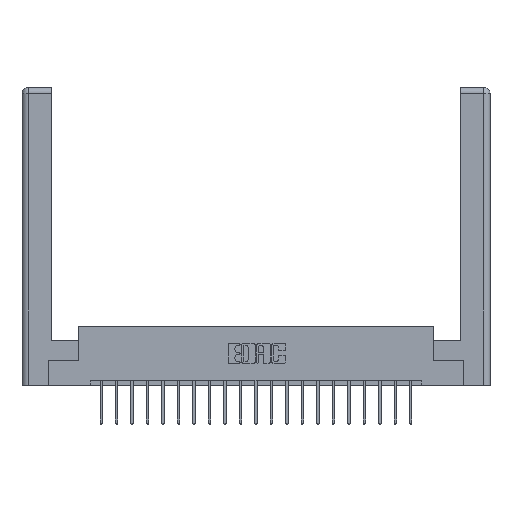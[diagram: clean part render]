
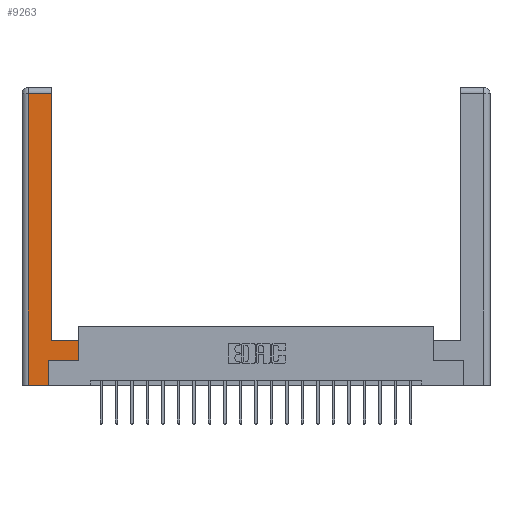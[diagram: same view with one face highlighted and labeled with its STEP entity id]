
A CAD part, top view. The second image highlights one B-rep face of the part: STEP entity #9263.
In plain terms, the highlighted planar face has unit normal (0, 0, 1).
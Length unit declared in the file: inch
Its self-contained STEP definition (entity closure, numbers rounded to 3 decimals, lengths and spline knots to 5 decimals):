
#172 = VECTOR ( 'NONE', #19106, 39.37008 ) ;
#198 = VECTOR ( 'NONE', #21235, 39.37008 ) ;
#546 = CARTESIAN_POINT ( 'NONE',  ( 0.565, 0.45, 0. ) ) ;
#695 = VECTOR ( 'NONE', #6751, 39.37008 ) ;
#976 = CARTESIAN_POINT ( 'NONE',  ( 0.265, 0., 0. ) ) ;
#1071 = CARTESIAN_POINT ( 'NONE',  ( 0.265, 0.245, 0. ) ) ;
#1499 = ORIENTED_EDGE ( 'NONE', *, *, #1673, .T. ) ;
#1673 = EDGE_CURVE ( 'NONE', #5320, #14640, #13986, .T. ) ;
#1814 = ORIENTED_EDGE ( 'NONE', *, *, #2555, .T. ) ;
#2351 = CARTESIAN_POINT ( 'NONE',  ( 0.0615, 0., 0. ) ) ;
#2555 = EDGE_CURVE ( 'NONE', #11462, #7162, #8593, .T. ) ;
#3026 = ORIENTED_EDGE ( 'NONE', *, *, #10543, .T. ) ;
#3735 = LINE ( 'NONE', #19542, #17870 ) ;
#4476 = DIRECTION ( 'NONE',  ( 1., 0., 0. ) ) ;
#5158 = CARTESIAN_POINT ( 'NONE',  ( 0.295, 0.45, 0. ) ) ;
#5320 = VERTEX_POINT ( 'NONE', #20268 ) ;
#5888 = PLANE ( 'NONE',  #10201 ) ;
#6183 = FACE_OUTER_BOUND ( 'NONE', #14101, .T. ) ;
#6222 = EDGE_CURVE ( 'NONE', #7162, #16424, #13292, .T. ) ;
#6457 = VERTEX_POINT ( 'NONE', #5158 ) ;
#6659 = CARTESIAN_POINT ( 'NONE',  ( 0.0615, 0., 0. ) ) ;
#6751 = DIRECTION ( 'NONE',  ( 0., 1., 0. ) ) ;
#7162 = VERTEX_POINT ( 'NONE', #16724 ) ;
#7214 = VECTOR ( 'NONE', #15144, 39.37008 ) ;
#7555 = EDGE_CURVE ( 'NONE', #14640, #18756, #17648, .T. ) ;
#8104 = CARTESIAN_POINT ( 'NONE',  ( 0.565, 0.245, 0. ) ) ;
#8262 = LINE ( 'NONE', #21113, #16854 ) ;
#8593 = LINE ( 'NONE', #1071, #172 ) ;
#8949 = CARTESIAN_POINT ( 'NONE',  ( 0.0615, 2.94, 0. ) ) ;
#9033 = DIRECTION ( 'NONE',  ( -1., 0., 0. ) ) ;
#9263 = ADVANCED_FACE ( 'NONE', ( #6183 ), #5888, .F. ) ;
#10069 = VECTOR ( 'NONE', #20673, 39.37008 ) ;
#10118 = CARTESIAN_POINT ( 'NONE',  ( 0.565, 0.45, 0. ) ) ;
#10201 = AXIS2_PLACEMENT_3D ( 'NONE', #19228, #20625, #9033 ) ;
#10543 = EDGE_CURVE ( 'NONE', #18756, #11462, #8262, .T. ) ;
#11230 = ORIENTED_EDGE ( 'NONE', *, *, #15108, .T. ) ;
#11462 = VERTEX_POINT ( 'NONE', #976 ) ;
#11577 = VERTEX_POINT ( 'NONE', #546 ) ;
#13292 = LINE ( 'NONE', #14527, #20068 ) ;
#13296 = CARTESIAN_POINT ( 'NONE',  ( 0.0615, 2.94, 0. ) ) ;
#13986 = LINE ( 'NONE', #8949, #10069 ) ;
#14101 = EDGE_LOOP ( 'NONE', ( #11230, #1499, #19694, #3026, #1814, #16645, #19634, #16301 ) ) ;
#14115 = LINE ( 'NONE', #16231, #198 ) ;
#14527 = CARTESIAN_POINT ( 'NONE',  ( 0.565, 0.245, 0. ) ) ;
#14640 = VERTEX_POINT ( 'NONE', #13296 ) ;
#15108 = EDGE_CURVE ( 'NONE', #6457, #5320, #3735, .T. ) ;
#15144 = DIRECTION ( 'NONE',  ( 0., -1., 0. ) ) ;
#16231 = CARTESIAN_POINT ( 'NONE',  ( 0.295, 0.45, 0. ) ) ;
#16301 = ORIENTED_EDGE ( 'NONE', *, *, #17587, .T. ) ;
#16424 = VERTEX_POINT ( 'NONE', #8104 ) ;
#16425 = LINE ( 'NONE', #10118, #695 ) ;
#16645 = ORIENTED_EDGE ( 'NONE', *, *, #6222, .T. ) ;
#16724 = CARTESIAN_POINT ( 'NONE',  ( 0.265, 0.245, 0. ) ) ;
#16854 = VECTOR ( 'NONE', #4476, 39.37008 ) ;
#17587 = EDGE_CURVE ( 'NONE', #11577, #6457, #14115, .T. ) ;
#17648 = LINE ( 'NONE', #6659, #7214 ) ;
#17870 = VECTOR ( 'NONE', #19756, 39.37008 ) ;
#18756 = VERTEX_POINT ( 'NONE', #2351 ) ;
#19106 = DIRECTION ( 'NONE',  ( 0., 1., 0. ) ) ;
#19228 = CARTESIAN_POINT ( 'NONE',  ( 0., 0., 0. ) ) ;
#19542 = CARTESIAN_POINT ( 'NONE',  ( 0.295, 3., 0. ) ) ;
#19634 = ORIENTED_EDGE ( 'NONE', *, *, #20940, .T. ) ;
#19694 = ORIENTED_EDGE ( 'NONE', *, *, #7555, .T. ) ;
#19756 = DIRECTION ( 'NONE',  ( 0., 1., 0. ) ) ;
#20068 = VECTOR ( 'NONE', #21224, 39.37008 ) ;
#20268 = CARTESIAN_POINT ( 'NONE',  ( 0.295, 2.94, 0. ) ) ;
#20625 = DIRECTION ( 'NONE',  ( 0., 0., -1. ) ) ;
#20673 = DIRECTION ( 'NONE',  ( -1., 0., 0. ) ) ;
#20940 = EDGE_CURVE ( 'NONE', #16424, #11577, #16425, .T. ) ;
#21113 = CARTESIAN_POINT ( 'NONE',  ( 0.265, 0., 0. ) ) ;
#21224 = DIRECTION ( 'NONE',  ( 1., 0., 0. ) ) ;
#21235 = DIRECTION ( 'NONE',  ( -1., 0., 0. ) ) ;
